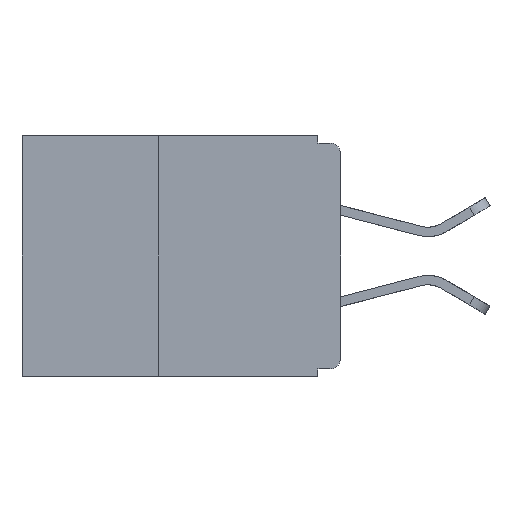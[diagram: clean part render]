
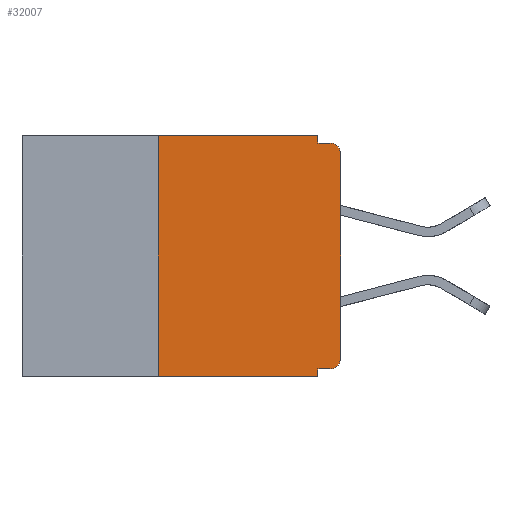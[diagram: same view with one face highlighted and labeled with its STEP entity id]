
A CAD part, left-side view. The second image highlights one B-rep face of the part: STEP entity #32007.
In plain terms, the highlighted planar face has unit normal (-1, 0, 0).
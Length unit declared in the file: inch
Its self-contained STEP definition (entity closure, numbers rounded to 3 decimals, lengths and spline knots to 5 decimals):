
#139 = PLANE ( 'NONE',  #15142 ) ;
#518 = DIRECTION ( 'NONE',  ( 0., 0., 1. ) ) ;
#843 = EDGE_CURVE ( 'NONE', #13209, #25392, #32031, .T. ) ;
#1938 = AXIS2_PLACEMENT_3D ( 'NONE', #25164, #9883, #27685 ) ;
#1981 = CARTESIAN_POINT ( 'NONE',  ( 0., 0.25, 0. ) ) ;
#2409 = ORIENTED_EDGE ( 'NONE', *, *, #4398, .F. ) ;
#2718 = VERTEX_POINT ( 'NONE', #15137 ) ;
#3149 = DIRECTION ( 'NONE',  ( 0., 0., -1. ) ) ;
#3717 = LINE ( 'NONE', #32381, #30054 ) ;
#4398 = EDGE_CURVE ( 'NONE', #22754, #31385, #31794, .T. ) ;
#4930 = ORIENTED_EDGE ( 'NONE', *, *, #31156, .F. ) ;
#5130 = EDGE_CURVE ( 'NONE', #14499, #2718, #15582, .T. ) ;
#5357 = DIRECTION ( 'NONE',  ( 1., 0., 0. ) ) ;
#6063 = CARTESIAN_POINT ( 'NONE',  ( 0., 0.25, -0.33 ) ) ;
#6425 = CARTESIAN_POINT ( 'NONE',  ( 0., 0.031, -0.01 ) ) ;
#7557 = DIRECTION ( 'NONE',  ( 0., 0., -1. ) ) ;
#8023 = LINE ( 'NONE', #22854, #14099 ) ;
#8979 = EDGE_CURVE ( 'NONE', #26326, #32676, #23665, .T. ) ;
#9362 = EDGE_CURVE ( 'NONE', #25392, #28141, #31870, .T. ) ;
#9883 = DIRECTION ( 'NONE',  ( -1., 0., 0. ) ) ;
#9895 = VECTOR ( 'NONE', #32018, 39.37008 ) ;
#10102 = VECTOR ( 'NONE', #3149, 39.37008 ) ;
#10585 = CARTESIAN_POINT ( 'NONE',  ( 0., 0.437, -0.33 ) ) ;
#11044 = CARTESIAN_POINT ( 'NONE',  ( 0., 0.031, 0. ) ) ;
#11143 = CARTESIAN_POINT ( 'NONE',  ( 0., 0.015, -0.32 ) ) ;
#11560 = ORIENTED_EDGE ( 'NONE', *, *, #9362, .T. ) ;
#11825 = CARTESIAN_POINT ( 'NONE',  ( 0., 0.25, -0.33 ) ) ;
#13209 = VERTEX_POINT ( 'NONE', #11143 ) ;
#13333 = LINE ( 'NONE', #10585, #27599 ) ;
#13420 = CARTESIAN_POINT ( 'NONE',  ( 0., 0., -0.305 ) ) ;
#13932 = ORIENTED_EDGE ( 'NONE', *, *, #27240, .F. ) ;
#14099 = VECTOR ( 'NONE', #7557, 39.37008 ) ;
#14276 = DIRECTION ( 'NONE',  ( 0., 0., -1. ) ) ;
#14499 = VERTEX_POINT ( 'NONE', #6425 ) ;
#14912 = VERTEX_POINT ( 'NONE', #6063 ) ;
#15137 = CARTESIAN_POINT ( 'NONE',  ( 0., 0.015, -0.01 ) ) ;
#15142 = AXIS2_PLACEMENT_3D ( 'NONE', #20646, #5357, #23258 ) ;
#15214 = ORIENTED_EDGE ( 'NONE', *, *, #20902, .F. ) ;
#15582 = LINE ( 'NONE', #32323, #28253 ) ;
#15980 = CARTESIAN_POINT ( 'NONE',  ( 0., 0., 0. ) ) ;
#16087 = DIRECTION ( 'NONE',  ( -1., 0., 0. ) ) ;
#16344 = CARTESIAN_POINT ( 'NONE',  ( 0., 0.015, -0.305 ) ) ;
#16749 = LINE ( 'NONE', #11825, #9895 ) ;
#17470 = ORIENTED_EDGE ( 'NONE', *, *, #29373, .T. ) ;
#18345 = ORIENTED_EDGE ( 'NONE', *, *, #843, .T. ) ;
#18515 = VECTOR ( 'NONE', #518, 39.37008 ) ;
#18575 = CARTESIAN_POINT ( 'NONE',  ( 0., 0.031, -0.33 ) ) ;
#19578 = CARTESIAN_POINT ( 'NONE',  ( 0., 0.437, 0. ) ) ;
#20646 = CARTESIAN_POINT ( 'NONE',  ( 0., 0.437, 0. ) ) ;
#20837 = ORIENTED_EDGE ( 'NONE', *, *, #8979, .F. ) ;
#20902 = EDGE_CURVE ( 'NONE', #14912, #22754, #16749, .T. ) ;
#21267 = CARTESIAN_POINT ( 'NONE',  ( 0., 0.031, -0.33 ) ) ;
#21584 = FACE_OUTER_BOUND ( 'NONE', #24256, .T. ) ;
#22754 = VERTEX_POINT ( 'NONE', #1981 ) ;
#22854 = CARTESIAN_POINT ( 'NONE',  ( 0., 0.031, 0. ) ) ;
#23201 = AXIS2_PLACEMENT_3D ( 'NONE', #16344, #16087, #14276 ) ;
#23258 = DIRECTION ( 'NONE',  ( 0., 0., -1. ) ) ;
#23299 = DIRECTION ( 'NONE',  ( 0., -1., 0. ) ) ;
#23553 = CIRCLE ( 'NONE', #1938, 0.015 ) ;
#23665 = LINE ( 'NONE', #18575, #10102 ) ;
#23711 = ORIENTED_EDGE ( 'NONE', *, *, #31723, .T. ) ;
#24256 = EDGE_LOOP ( 'NONE', ( #11560, #23711, #26910, #4930, #2409, #15214, #17470, #20837, #13932, #18345 ) ) ;
#24983 = DIRECTION ( 'NONE',  ( 0., 1., 0. ) ) ;
#25164 = CARTESIAN_POINT ( 'NONE',  ( 0., 0.015, -0.025 ) ) ;
#25392 = VERTEX_POINT ( 'NONE', #13420 ) ;
#26326 = VERTEX_POINT ( 'NONE', #28447 ) ;
#26910 = ORIENTED_EDGE ( 'NONE', *, *, #5130, .F. ) ;
#27240 = EDGE_CURVE ( 'NONE', #13209, #26326, #3717, .T. ) ;
#27340 = DIRECTION ( 'NONE',  ( 0., -1., 0. ) ) ;
#27599 = VECTOR ( 'NONE', #23299, 39.37008 ) ;
#27685 = DIRECTION ( 'NONE',  ( 0., 0., -1. ) ) ;
#28141 = VERTEX_POINT ( 'NONE', #28454 ) ;
#28253 = VECTOR ( 'NONE', #27340, 39.37008 ) ;
#28447 = CARTESIAN_POINT ( 'NONE',  ( 0., 0.031, -0.32 ) ) ;
#28454 = CARTESIAN_POINT ( 'NONE',  ( 0., 0., -0.025 ) ) ;
#29373 = EDGE_CURVE ( 'NONE', #14912, #32676, #13333, .T. ) ;
#29474 = VECTOR ( 'NONE', #32049, 39.37008 ) ;
#30054 = VECTOR ( 'NONE', #24983, 39.37008 ) ;
#31156 = EDGE_CURVE ( 'NONE', #31385, #14499, #8023, .T. ) ;
#31385 = VERTEX_POINT ( 'NONE', #11044 ) ;
#31723 = EDGE_CURVE ( 'NONE', #28141, #2718, #23553, .T. ) ;
#31794 = LINE ( 'NONE', #19578, #29474 ) ;
#31870 = LINE ( 'NONE', #15980, #18515 ) ;
#32007 = ADVANCED_FACE ( 'NONE', ( #21584 ), #139, .F. ) ;
#32018 = DIRECTION ( 'NONE',  ( 0., 0., 1. ) ) ;
#32031 = CIRCLE ( 'NONE', #23201, 0.015 ) ;
#32049 = DIRECTION ( 'NONE',  ( 0., -1., 0. ) ) ;
#32323 = CARTESIAN_POINT ( 'NONE',  ( 0., 0., -0.01 ) ) ;
#32381 = CARTESIAN_POINT ( 'NONE',  ( 0., 0., -0.32 ) ) ;
#32676 = VERTEX_POINT ( 'NONE', #21267 ) ;
